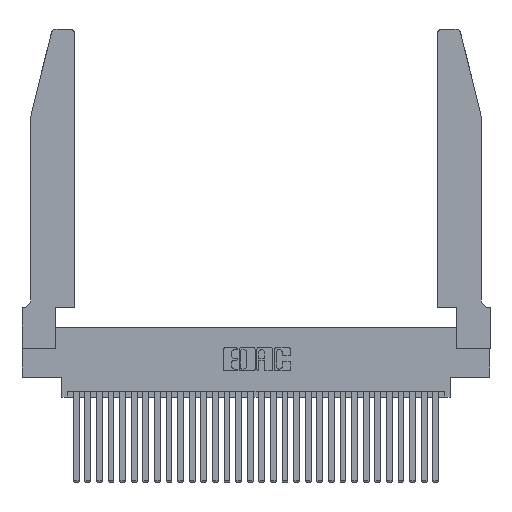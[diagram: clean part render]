
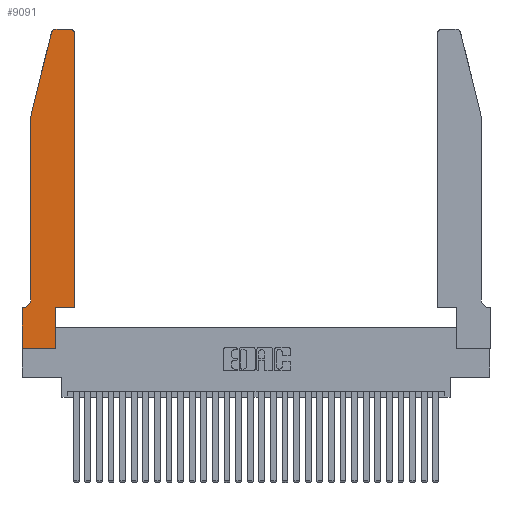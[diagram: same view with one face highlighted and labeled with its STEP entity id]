
A CAD part, top view. The second image highlights one B-rep face of the part: STEP entity #9091.
In plain terms, the highlighted planar face has unit normal (0, 0, 1).
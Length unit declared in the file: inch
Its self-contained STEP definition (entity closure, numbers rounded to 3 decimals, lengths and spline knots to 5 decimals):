
#310 = DIRECTION ( 'NONE',  ( 0., 1., 0. ) ) ;
#1364 = CARTESIAN_POINT ( 'NONE',  ( 0.25487, 2.72718, 0.37 ) ) ;
#1595 = VECTOR ( 'NONE', #3350, 39.37008 ) ;
#1813 = EDGE_CURVE ( 'NONE', #2135, #20611, #22931, .T. ) ;
#2063 = CARTESIAN_POINT ( 'NONE',  ( 0.0755, 2., 0.37 ) ) ;
#2135 = VERTEX_POINT ( 'NONE', #7799 ) ;
#2448 = DIRECTION ( 'NONE',  ( 0., -1., 0. ) ) ;
#2783 = VERTEX_POINT ( 'NONE', #29888 ) ;
#3181 = ORIENTED_EDGE ( 'NONE', *, *, #1813, .T. ) ;
#3350 = DIRECTION ( 'NONE',  ( -1., 0., 0. ) ) ;
#3388 = CARTESIAN_POINT ( 'NONE',  ( 0.4205, 2.72, 0.37 ) ) ;
#4371 = ORIENTED_EDGE ( 'NONE', *, *, #27125, .T. ) ;
#4516 = CARTESIAN_POINT ( 'NONE',  ( 0.2865, 0.35, 0.37 ) ) ;
#4810 = ORIENTED_EDGE ( 'NONE', *, *, #12557, .T. ) ;
#5448 = CARTESIAN_POINT ( 'NONE',  ( 0.0755, 0.42, 0.37 ) ) ;
#5560 = EDGE_CURVE ( 'NONE', #21400, #26287, #14442, .T. ) ;
#5661 = CARTESIAN_POINT ( 'NONE',  ( 0., 0.35, 0.37 ) ) ;
#5730 = VERTEX_POINT ( 'NONE', #21055 ) ;
#5857 = DIRECTION ( 'NONE',  ( 1., 0., 0. ) ) ;
#6212 = LINE ( 'NONE', #2063, #23904 ) ;
#6705 = DIRECTION ( 'NONE',  ( 1., 0., 0. ) ) ;
#7272 = CARTESIAN_POINT ( 'NONE',  ( 0.0755, 2., 0.37 ) ) ;
#7328 = VECTOR ( 'NONE', #16556, 39.37008 ) ;
#7799 = CARTESIAN_POINT ( 'NONE',  ( 0.2865, 0.35, 0.37 ) ) ;
#8087 = LINE ( 'NONE', #20279, #1595 ) ;
#8418 = DIRECTION ( 'NONE',  ( -1., 0., 0. ) ) ;
#8749 = VERTEX_POINT ( 'NONE', #5448 ) ;
#8906 = CIRCLE ( 'NONE', #24911, 0.03 ) ;
#8982 = VERTEX_POINT ( 'NONE', #1364 ) ;
#9008 = CARTESIAN_POINT ( 'NONE',  ( 0., 0., 0.37 ) ) ;
#9091 = ADVANCED_FACE ( 'NONE', ( #22453 ), #18729, .T. ) ;
#9560 = VERTEX_POINT ( 'NONE', #22903 ) ;
#10122 = EDGE_CURVE ( 'NONE', #5730, #26444, #8087, .T. ) ;
#10210 = LINE ( 'NONE', #9008, #22244 ) ;
#10578 = AXIS2_PLACEMENT_3D ( 'NONE', #12893, #29599, #15287 ) ;
#10902 = VECTOR ( 'NONE', #2448, 39.37008 ) ;
#11188 = ORIENTED_EDGE ( 'NONE', *, *, #19288, .T. ) ;
#11467 = DIRECTION ( 'NONE',  ( 1., 0., 0. ) ) ;
#11929 = AXIS2_PLACEMENT_3D ( 'NONE', #27447, #13114, #29813 ) ;
#12557 = EDGE_CURVE ( 'NONE', #26444, #8982, #26766, .T. ) ;
#12893 = CARTESIAN_POINT ( 'NONE',  ( 0.284, 2.72, 0.37 ) ) ;
#13033 = LINE ( 'NONE', #4516, #7328 ) ;
#13114 = DIRECTION ( 'NONE',  ( 0., 0., -1. ) ) ;
#13375 = VECTOR ( 'NONE', #25805, 39.37008 ) ;
#13540 = CARTESIAN_POINT ( 'NONE',  ( 0.0055, 0.35, 0.37 ) ) ;
#14114 = LINE ( 'NONE', #21111, #13375 ) ;
#14442 = LINE ( 'NONE', #15606, #25677 ) ;
#14597 = ORIENTED_EDGE ( 'NONE', *, *, #16617, .T. ) ;
#15105 = CARTESIAN_POINT ( 'NONE',  ( 0.0755, 2., 0.37 ) ) ;
#15217 = LINE ( 'NONE', #17300, #20871 ) ;
#15285 = CIRCLE ( 'NONE', #11929, 0.07 ) ;
#15287 = DIRECTION ( 'NONE',  ( 1., 0., 0. ) ) ;
#15445 = EDGE_CURVE ( 'NONE', #25610, #8749, #29981, .T. ) ;
#15606 = CARTESIAN_POINT ( 'NONE',  ( 0.0755, 0.35, 0.37 ) ) ;
#15693 = ORIENTED_EDGE ( 'NONE', *, *, #17634, .T. ) ;
#16530 = VECTOR ( 'NONE', #28273, 39.37008 ) ;
#16556 = DIRECTION ( 'NONE',  ( 0., 1., 0. ) ) ;
#16617 = EDGE_CURVE ( 'NONE', #9560, #5730, #8906, .T. ) ;
#17300 = CARTESIAN_POINT ( 'NONE',  ( 0.4505, 0.35, 0.37 ) ) ;
#17634 = EDGE_CURVE ( 'NONE', #2783, #2135, #13033, .T. ) ;
#18041 = ORIENTED_EDGE ( 'NONE', *, *, #10122, .T. ) ;
#18729 = PLANE ( 'NONE',  #20981 ) ;
#19015 = EDGE_CURVE ( 'NONE', #26287, #30132, #14114, .T. ) ;
#19288 = EDGE_CURVE ( 'NONE', #20611, #9560, #15217, .T. ) ;
#20279 = CARTESIAN_POINT ( 'NONE',  ( 0.2605, 2.75, 0.37 ) ) ;
#20321 = DIRECTION ( 'NONE',  ( 0., 0., 1. ) ) ;
#20611 = VERTEX_POINT ( 'NONE', #22258 ) ;
#20871 = VECTOR ( 'NONE', #310, 39.37008 ) ;
#20981 = AXIS2_PLACEMENT_3D ( 'NONE', #28216, #21142, #6705 ) ;
#21055 = CARTESIAN_POINT ( 'NONE',  ( 0.4205, 2.75, 0.37 ) ) ;
#21111 = CARTESIAN_POINT ( 'NONE',  ( 0., 0., 0.37 ) ) ;
#21142 = DIRECTION ( 'NONE',  ( 0., 0., 1. ) ) ;
#21400 = VERTEX_POINT ( 'NONE', #13540 ) ;
#22244 = VECTOR ( 'NONE', #11467, 39.37008 ) ;
#22258 = CARTESIAN_POINT ( 'NONE',  ( 0.4505, 0.35, 0.37 ) ) ;
#22453 = FACE_OUTER_BOUND ( 'NONE', #27324, .T. ) ;
#22903 = CARTESIAN_POINT ( 'NONE',  ( 0.4505, 2.72, 0.37 ) ) ;
#22931 = LINE ( 'NONE', #30552, #16530 ) ;
#23226 = ORIENTED_EDGE ( 'NONE', *, *, #19015, .T. ) ;
#23904 = VECTOR ( 'NONE', #28570, 39.37008 ) ;
#24381 = EDGE_CURVE ( 'NONE', #8749, #21400, #15285, .T. ) ;
#24911 = AXIS2_PLACEMENT_3D ( 'NONE', #3388, #20321, #5857 ) ;
#25610 = VERTEX_POINT ( 'NONE', #15105 ) ;
#25677 = VECTOR ( 'NONE', #8418, 39.37008 ) ;
#25729 = CARTESIAN_POINT ( 'NONE',  ( 0., 0., 0.37 ) ) ;
#25805 = DIRECTION ( 'NONE',  ( 0., -1., 0. ) ) ;
#26287 = VERTEX_POINT ( 'NONE', #5661 ) ;
#26444 = VERTEX_POINT ( 'NONE', #30203 ) ;
#26658 = ORIENTED_EDGE ( 'NONE', *, *, #24381, .T. ) ;
#26766 = CIRCLE ( 'NONE', #10578, 0.03 ) ;
#27125 = EDGE_CURVE ( 'NONE', #30132, #2783, #10210, .T. ) ;
#27324 = EDGE_LOOP ( 'NONE', ( #18041, #4810, #31056, #29244, #26658, #28148, #23226, #4371, #15693, #3181, #11188, #14597 ) ) ;
#27447 = CARTESIAN_POINT ( 'NONE',  ( 0.0055, 0.42, 0.37 ) ) ;
#28148 = ORIENTED_EDGE ( 'NONE', *, *, #5560, .T. ) ;
#28216 = CARTESIAN_POINT ( 'NONE',  ( 0., 0.35, 0.37 ) ) ;
#28273 = DIRECTION ( 'NONE',  ( 1., 0., 0. ) ) ;
#28570 = DIRECTION ( 'NONE',  ( -0.239, -0.971, 0. ) ) ;
#28933 = EDGE_CURVE ( 'NONE', #8982, #25610, #6212, .T. ) ;
#29244 = ORIENTED_EDGE ( 'NONE', *, *, #15445, .T. ) ;
#29599 = DIRECTION ( 'NONE',  ( 0., 0., 1. ) ) ;
#29813 = DIRECTION ( 'NONE',  ( -1., 0., 0. ) ) ;
#29888 = CARTESIAN_POINT ( 'NONE',  ( 0.2865, 0., 0.37 ) ) ;
#29981 = LINE ( 'NONE', #7272, #10902 ) ;
#30132 = VERTEX_POINT ( 'NONE', #25729 ) ;
#30203 = CARTESIAN_POINT ( 'NONE',  ( 0.284, 2.75, 0.37 ) ) ;
#30552 = CARTESIAN_POINT ( 'NONE',  ( 0.4505, 0.35, 0.37 ) ) ;
#31056 = ORIENTED_EDGE ( 'NONE', *, *, #28933, .T. ) ;
